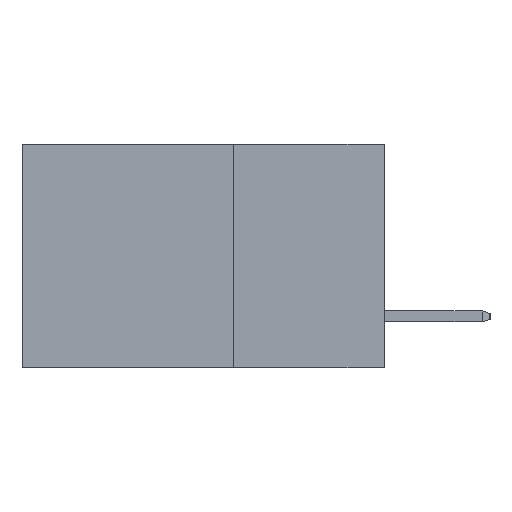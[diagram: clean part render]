
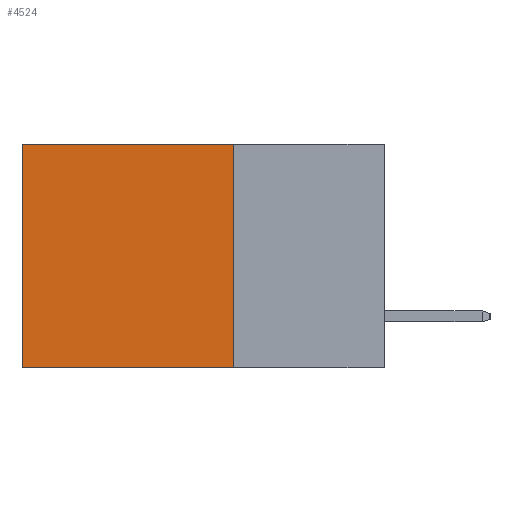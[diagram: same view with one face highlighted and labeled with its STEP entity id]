
A CAD part, left-side view. The second image highlights one B-rep face of the part: STEP entity #4524.
In plain terms, the highlighted planar face has unit normal (-1, 0, 0).
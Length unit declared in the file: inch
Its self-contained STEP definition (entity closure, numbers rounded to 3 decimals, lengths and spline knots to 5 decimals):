
#300 = CARTESIAN_POINT ( 'NONE',  ( 0.2615, 0.6, -0.37 ) ) ;
#330 = ORIENTED_EDGE ( 'NONE', *, *, #14494, .F. ) ;
#561 = CARTESIAN_POINT ( 'NONE',  ( 0.2615, 0.25, -0.37 ) ) ;
#741 = ORIENTED_EDGE ( 'NONE', *, *, #4102, .T. ) ;
#1085 = LINE ( 'NONE', #300, #8550 ) ;
#2173 = ORIENTED_EDGE ( 'NONE', *, *, #12656, .T. ) ;
#2567 = PLANE ( 'NONE',  #15163 ) ;
#2867 = LINE ( 'NONE', #10782, #12542 ) ;
#3113 = DIRECTION ( 'NONE',  ( 0., 0., -1. ) ) ;
#3853 = CARTESIAN_POINT ( 'NONE',  ( 0.2615, 0.25, -0.37 ) ) ;
#4102 = EDGE_CURVE ( 'NONE', #12244, #8942, #1085, .T. ) ;
#4524 = ADVANCED_FACE ( 'NONE', ( #11145 ), #2567, .F. ) ;
#4806 = EDGE_LOOP ( 'NONE', ( #741, #330, #11617, #2173 ) ) ;
#5620 = CARTESIAN_POINT ( 'NONE',  ( 0.2615, 0.25, 0. ) ) ;
#6213 = CARTESIAN_POINT ( 'NONE',  ( 0.2615, 0.6, -0.37 ) ) ;
#6354 = DIRECTION ( 'NONE',  ( 0., 0., -1. ) ) ;
#6596 = DIRECTION ( 'NONE',  ( 0., 0., -1. ) ) ;
#6885 = VECTOR ( 'NONE', #9458, 39.37008 ) ;
#8550 = VECTOR ( 'NONE', #6596, 39.37008 ) ;
#8942 = VERTEX_POINT ( 'NONE', #6213 ) ;
#9458 = DIRECTION ( 'NONE',  ( 0., 1., 0. ) ) ;
#10286 = LINE ( 'NONE', #5620, #6885 ) ;
#10782 = CARTESIAN_POINT ( 'NONE',  ( 0.2615, 0.25, -0.37 ) ) ;
#11076 = CARTESIAN_POINT ( 'NONE',  ( 0.2615, 0.25, -0.37 ) ) ;
#11145 = FACE_OUTER_BOUND ( 'NONE', #4806, .T. ) ;
#11295 = VERTEX_POINT ( 'NONE', #11076 ) ;
#11617 = ORIENTED_EDGE ( 'NONE', *, *, #12636, .F. ) ;
#12244 = VERTEX_POINT ( 'NONE', #16108 ) ;
#12542 = VECTOR ( 'NONE', #13320, 39.37008 ) ;
#12636 = EDGE_CURVE ( 'NONE', #14560, #11295, #14025, .T. ) ;
#12656 = EDGE_CURVE ( 'NONE', #14560, #12244, #10286, .T. ) ;
#13320 = DIRECTION ( 'NONE',  ( 0., 1., 0. ) ) ;
#13626 = VECTOR ( 'NONE', #3113, 39.37008 ) ;
#13948 = DIRECTION ( 'NONE',  ( 1., 0., 0. ) ) ;
#14025 = LINE ( 'NONE', #561, #13626 ) ;
#14494 = EDGE_CURVE ( 'NONE', #11295, #8942, #2867, .T. ) ;
#14560 = VERTEX_POINT ( 'NONE', #15924 ) ;
#15163 = AXIS2_PLACEMENT_3D ( 'NONE', #3853, #13948, #6354 ) ;
#15924 = CARTESIAN_POINT ( 'NONE',  ( 0.2615, 0.25, 0. ) ) ;
#16108 = CARTESIAN_POINT ( 'NONE',  ( 0.2615, 0.6, 0. ) ) ;
